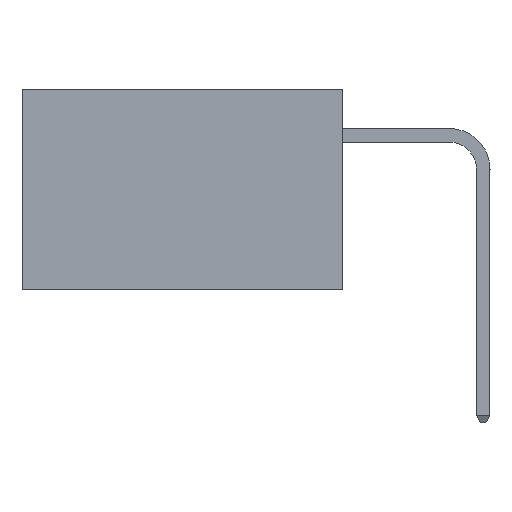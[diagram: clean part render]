
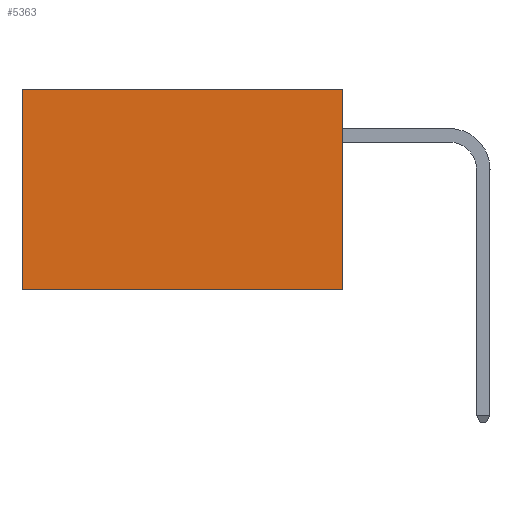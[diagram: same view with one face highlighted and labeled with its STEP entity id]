
A CAD part, left-side view. The second image highlights one B-rep face of the part: STEP entity #5363.
In plain terms, the highlighted planar face has unit normal (-1, 0, 0).
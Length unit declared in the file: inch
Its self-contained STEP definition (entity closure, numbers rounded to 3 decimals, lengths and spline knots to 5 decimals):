
#236 = LINE ( 'NONE', #14962, #16372 ) ;
#356 = DIRECTION ( 'NONE',  ( 0., 0., -1. ) ) ;
#1954 = CARTESIAN_POINT ( 'NONE',  ( 0.277, 0., 0. ) ) ;
#2505 = CARTESIAN_POINT ( 'NONE',  ( 0.277, 0., -0.37 ) ) ;
#2540 = CARTESIAN_POINT ( 'NONE',  ( 0.277, 0., 0. ) ) ;
#4517 = VECTOR ( 'NONE', #356, 39.37008 ) ;
#4709 = EDGE_CURVE ( 'NONE', #13155, #19340, #236, .T. ) ;
#5363 = ADVANCED_FACE ( 'NONE', ( #9028 ), #8297, .F. ) ;
#5474 = AXIS2_PLACEMENT_3D ( 'NONE', #8376, #8126, #8153 ) ;
#5769 = VECTOR ( 'NONE', #14161, 39.37008 ) ;
#6410 = VERTEX_POINT ( 'NONE', #16520 ) ;
#6701 = LINE ( 'NONE', #1954, #5769 ) ;
#6754 = ORIENTED_EDGE ( 'NONE', *, *, #4709, .F. ) ;
#8126 = DIRECTION ( 'NONE',  ( 1., 0., 0. ) ) ;
#8153 = DIRECTION ( 'NONE',  ( 0., 0., -1. ) ) ;
#8297 = PLANE ( 'NONE',  #5474 ) ;
#8376 = CARTESIAN_POINT ( 'NONE',  ( 0.277, 0., -0.37 ) ) ;
#8586 = LINE ( 'NONE', #18469, #4517 ) ;
#9028 = FACE_OUTER_BOUND ( 'NONE', #16401, .T. ) ;
#9333 = DIRECTION ( 'NONE',  ( 0., 1., 0. ) ) ;
#9923 = ORIENTED_EDGE ( 'NONE', *, *, #16186, .T. ) ;
#10819 = CARTESIAN_POINT ( 'NONE',  ( 0.277, 0., -0.37 ) ) ;
#10941 = VECTOR ( 'NONE', #9333, 39.37008 ) ;
#11406 = ORIENTED_EDGE ( 'NONE', *, *, #15478, .T. ) ;
#12861 = EDGE_CURVE ( 'NONE', #19340, #6410, #18953, .T. ) ;
#13155 = VERTEX_POINT ( 'NONE', #2540 ) ;
#13967 = ORIENTED_EDGE ( 'NONE', *, *, #12861, .F. ) ;
#14161 = DIRECTION ( 'NONE',  ( 0., 1., 0. ) ) ;
#14879 = CARTESIAN_POINT ( 'NONE',  ( 0.277, 0.59, 0. ) ) ;
#14962 = CARTESIAN_POINT ( 'NONE',  ( 0.277, 0., -0.37 ) ) ;
#15478 = EDGE_CURVE ( 'NONE', #13155, #15801, #6701, .T. ) ;
#15801 = VERTEX_POINT ( 'NONE', #14879 ) ;
#16186 = EDGE_CURVE ( 'NONE', #15801, #6410, #8586, .T. ) ;
#16372 = VECTOR ( 'NONE', #18988, 39.37008 ) ;
#16401 = EDGE_LOOP ( 'NONE', ( #9923, #13967, #6754, #11406 ) ) ;
#16520 = CARTESIAN_POINT ( 'NONE',  ( 0.277, 0.59, -0.37 ) ) ;
#18469 = CARTESIAN_POINT ( 'NONE',  ( 0.277, 0.59, -0.37 ) ) ;
#18953 = LINE ( 'NONE', #10819, #10941 ) ;
#18988 = DIRECTION ( 'NONE',  ( 0., 0., -1. ) ) ;
#19340 = VERTEX_POINT ( 'NONE', #2505 ) ;
